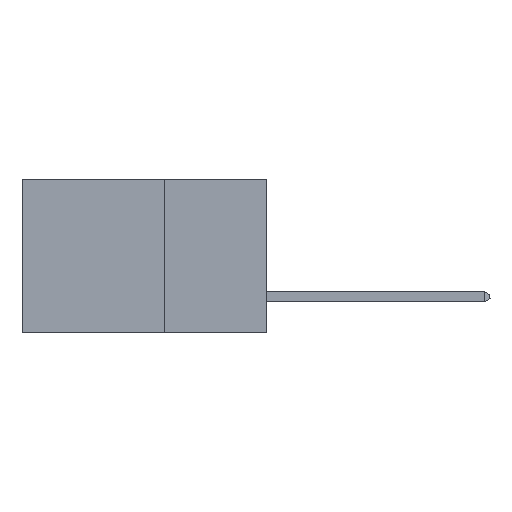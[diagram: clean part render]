
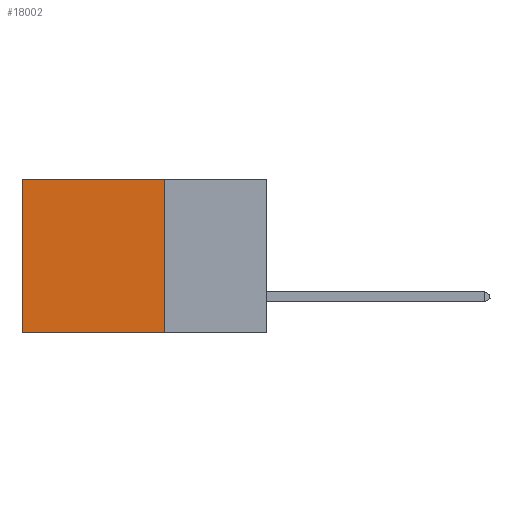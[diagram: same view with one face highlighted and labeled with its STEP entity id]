
A CAD part, left-side view. The second image highlights one B-rep face of the part: STEP entity #18002.
In plain terms, the highlighted planar face has unit normal (-1, 0, 0).
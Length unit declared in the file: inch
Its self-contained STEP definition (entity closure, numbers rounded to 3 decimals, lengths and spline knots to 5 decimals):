
#944 = VECTOR ( 'NONE', #15218, 39.37008 ) ;
#1423 = FACE_OUTER_BOUND ( 'NONE', #1435, .T. ) ;
#1435 = EDGE_LOOP ( 'NONE', ( #5402, #3791, #13756, #12755 ) ) ;
#1578 = LINE ( 'NONE', #7084, #8936 ) ;
#2144 = CARTESIAN_POINT ( 'NONE',  ( 0.2875, 0.25, -0.375 ) ) ;
#2418 = EDGE_CURVE ( 'NONE', #7038, #13953, #18536, .T. ) ;
#3442 = EDGE_CURVE ( 'NONE', #9095, #12101, #1578, .T. ) ;
#3791 = ORIENTED_EDGE ( 'NONE', *, *, #12061, .F. ) ;
#5402 = ORIENTED_EDGE ( 'NONE', *, *, #3442, .T. ) ;
#5550 = PLANE ( 'NONE',  #7238 ) ;
#6657 = VECTOR ( 'NONE', #16905, 39.37008 ) ;
#7021 = CARTESIAN_POINT ( 'NONE',  ( 0.2875, 0.25, -0.375 ) ) ;
#7038 = VERTEX_POINT ( 'NONE', #14434 ) ;
#7044 = DIRECTION ( 'NONE',  ( 0., 0., -1. ) ) ;
#7084 = CARTESIAN_POINT ( 'NONE',  ( 0.2875, 0.6, -0.375 ) ) ;
#7238 = AXIS2_PLACEMENT_3D ( 'NONE', #9985, #15984, #7044 ) ;
#8314 = LINE ( 'NONE', #2144, #944 ) ;
#8571 = CARTESIAN_POINT ( 'NONE',  ( 0.2875, 0.25, 0. ) ) ;
#8936 = VECTOR ( 'NONE', #17477, 39.37008 ) ;
#9095 = VERTEX_POINT ( 'NONE', #11123 ) ;
#9985 = CARTESIAN_POINT ( 'NONE',  ( 0.2875, 0.25, -0.375 ) ) ;
#9989 = VECTOR ( 'NONE', #16130, 39.37008 ) ;
#11123 = CARTESIAN_POINT ( 'NONE',  ( 0.2875, 0.6, 0. ) ) ;
#11189 = CARTESIAN_POINT ( 'NONE',  ( 0.2875, 0.25, -0.375 ) ) ;
#12061 = EDGE_CURVE ( 'NONE', #13953, #12101, #8314, .T. ) ;
#12101 = VERTEX_POINT ( 'NONE', #15783 ) ;
#12755 = ORIENTED_EDGE ( 'NONE', *, *, #15566, .T. ) ;
#13756 = ORIENTED_EDGE ( 'NONE', *, *, #2418, .F. ) ;
#13953 = VERTEX_POINT ( 'NONE', #7021 ) ;
#13973 = LINE ( 'NONE', #8571, #9989 ) ;
#14434 = CARTESIAN_POINT ( 'NONE',  ( 0.2875, 0.25, 0. ) ) ;
#15218 = DIRECTION ( 'NONE',  ( 0., 1., 0. ) ) ;
#15566 = EDGE_CURVE ( 'NONE', #7038, #9095, #13973, .T. ) ;
#15783 = CARTESIAN_POINT ( 'NONE',  ( 0.2875, 0.6, -0.375 ) ) ;
#15984 = DIRECTION ( 'NONE',  ( 1., 0., 0. ) ) ;
#16130 = DIRECTION ( 'NONE',  ( 0., 1., 0. ) ) ;
#16905 = DIRECTION ( 'NONE',  ( 0., 0., -1. ) ) ;
#17477 = DIRECTION ( 'NONE',  ( 0., 0., -1. ) ) ;
#18002 = ADVANCED_FACE ( 'NONE', ( #1423 ), #5550, .F. ) ;
#18536 = LINE ( 'NONE', #11189, #6657 ) ;
